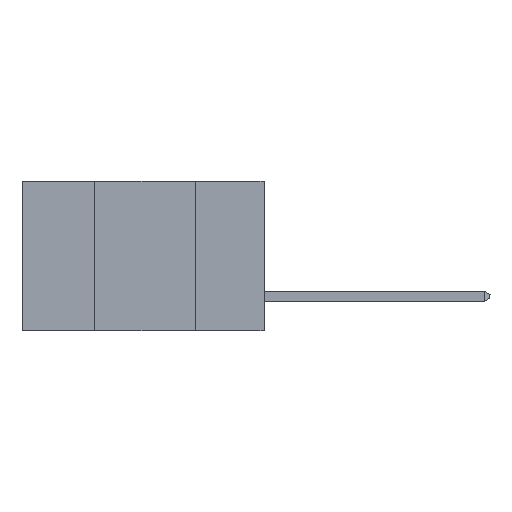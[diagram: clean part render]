
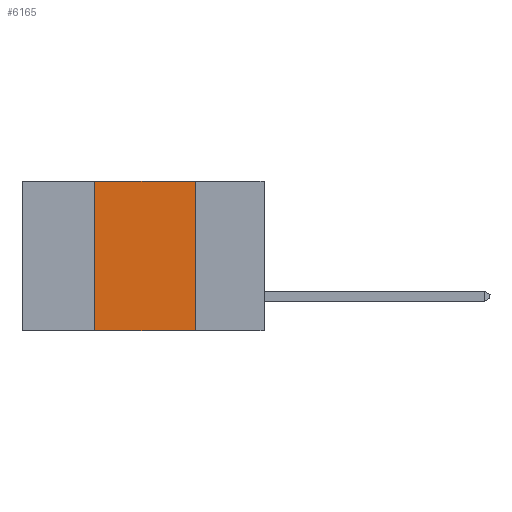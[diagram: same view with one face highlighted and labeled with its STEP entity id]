
A CAD part, left-side view. The second image highlights one B-rep face of the part: STEP entity #6165.
In plain terms, the highlighted planar face has unit normal (-1, 0, 0).
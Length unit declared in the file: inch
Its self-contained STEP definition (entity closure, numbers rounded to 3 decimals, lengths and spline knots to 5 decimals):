
#39 = VECTOR ( 'NONE', #16134, 39.37008 ) ;
#527 = LINE ( 'NONE', #5884, #39 ) ;
#1299 = VECTOR ( 'NONE', #2684, 39.37008 ) ;
#2684 = DIRECTION ( 'NONE',  ( 0., 0., 1. ) ) ;
#2829 = PLANE ( 'NONE',  #11934 ) ;
#2864 = EDGE_CURVE ( 'NONE', #7310, #15395, #15162, .T. ) ;
#2974 = FACE_OUTER_BOUND ( 'NONE', #3311, .T. ) ;
#3311 = EDGE_LOOP ( 'NONE', ( #7185, #3350, #8344, #6861 ) ) ;
#3350 = ORIENTED_EDGE ( 'NONE', *, *, #2864, .F. ) ;
#4288 = DIRECTION ( 'NONE',  ( 1., 0., 0. ) ) ;
#4565 = EDGE_CURVE ( 'NONE', #5001, #7310, #12995, .T. ) ;
#5001 = VERTEX_POINT ( 'NONE', #12327 ) ;
#5127 = EDGE_CURVE ( 'NONE', #5001, #12373, #527, .T. ) ;
#5785 = VECTOR ( 'NONE', #8124, 39.37008 ) ;
#5884 = CARTESIAN_POINT ( 'NONE',  ( 0., 0.6, -0.37 ) ) ;
#6165 = ADVANCED_FACE ( 'NONE', ( #2974 ), #2829, .F. ) ;
#6861 = ORIENTED_EDGE ( 'NONE', *, *, #5127, .T. ) ;
#7185 = ORIENTED_EDGE ( 'NONE', *, *, #17115, .F. ) ;
#7229 = DIRECTION ( 'NONE',  ( 0., 0., -1. ) ) ;
#7310 = VERTEX_POINT ( 'NONE', #18915 ) ;
#7311 = VECTOR ( 'NONE', #11975, 39.37008 ) ;
#8124 = DIRECTION ( 'NONE',  ( 0., 0., -1. ) ) ;
#8344 = ORIENTED_EDGE ( 'NONE', *, *, #4565, .F. ) ;
#11181 = CARTESIAN_POINT ( 'NONE',  ( 0., 0.6, 0. ) ) ;
#11934 = AXIS2_PLACEMENT_3D ( 'NONE', #11181, #4288, #7229 ) ;
#11975 = DIRECTION ( 'NONE',  ( 0., -1., 0. ) ) ;
#12327 = CARTESIAN_POINT ( 'NONE',  ( 0., 0.42, -0.37 ) ) ;
#12373 = VERTEX_POINT ( 'NONE', #13708 ) ;
#12631 = CARTESIAN_POINT ( 'NONE',  ( 0., 0.17, 0. ) ) ;
#12995 = LINE ( 'NONE', #15829, #1299 ) ;
#13312 = CARTESIAN_POINT ( 'NONE',  ( 0., 0.6, 0. ) ) ;
#13708 = CARTESIAN_POINT ( 'NONE',  ( 0., 0.17, -0.37 ) ) ;
#13927 = LINE ( 'NONE', #12631, #5785 ) ;
#14998 = CARTESIAN_POINT ( 'NONE',  ( 0., 0.17, 0. ) ) ;
#15162 = LINE ( 'NONE', #13312, #7311 ) ;
#15395 = VERTEX_POINT ( 'NONE', #14998 ) ;
#15829 = CARTESIAN_POINT ( 'NONE',  ( 0., 0.42, 0. ) ) ;
#16134 = DIRECTION ( 'NONE',  ( 0., -1., 0. ) ) ;
#17115 = EDGE_CURVE ( 'NONE', #15395, #12373, #13927, .T. ) ;
#18915 = CARTESIAN_POINT ( 'NONE',  ( 0., 0.42, 0. ) ) ;
